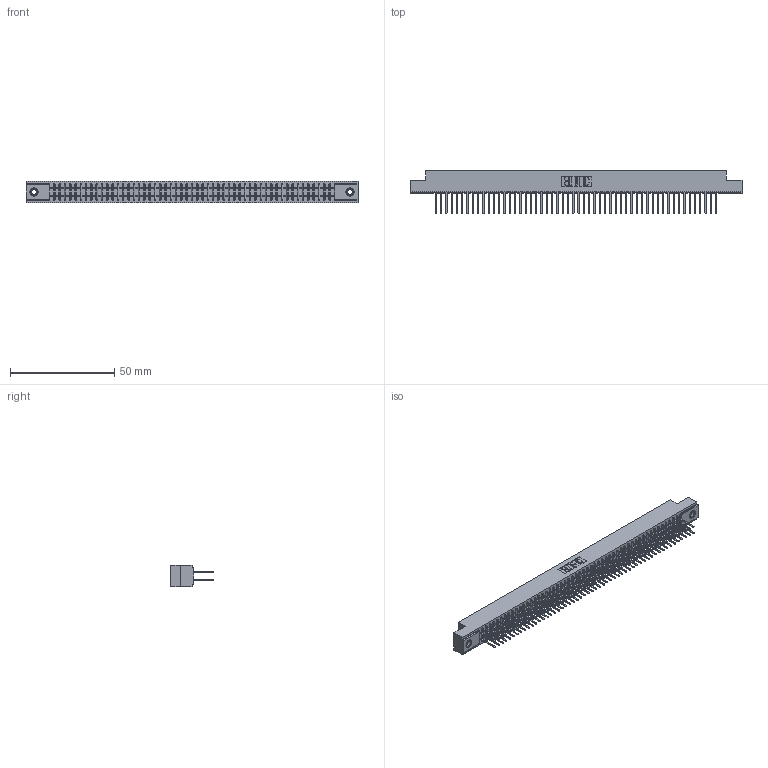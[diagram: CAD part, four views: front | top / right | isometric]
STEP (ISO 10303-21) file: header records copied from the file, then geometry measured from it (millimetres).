
FILE_DESCRIPTION (( 'STEP AP203' ), '1' );
FILE_NAME ('341-108-522-207.STEP', '2018-08-08T12:19:35', ( '' ), ( '' ), 'SwSTEP 2.0', 'SolidWorks 2016', '' );
FILE_SCHEMA (( 'CONFIG_CONTROL_DESIGN' ));
Products named in the file (4): 345-250-001_345-250-005-103; 341-108-522-207; 341 Part_.156 (3.96) Dia Mounting Holes; 341-292-001_341-292-122
Assembly tree (111 placements, depth 2):
  341-108-522-207
    341 Part_.156 (3.96) Dia Mounting Holes
    341-292-001_341-292-122  x108
    345-250-001_345-250-005-103  x2
Bounding box: 159.38 x 20.62 x 10.16 mm (x, y, z)
Volume: 11914.9 mm3; surface area: 22531.7 mm2
Topology: 111 solids, 111 shells, 7304 faces, 21134 edges, 13682 vertices
Faces by surface type: plane 4420, cylinder 2652, sphere 110, torus 110, cone 12
Entity records: 64938 total; most frequent: CARTESIAN_POINT 10777, ORIENTED_EDGE 10704, DIRECTION 10460, EDGE_CURVE 5352, VECTOR 4334, LINE 4334, VERTEX_POINT 3380, AXIS2_PLACEMENT_3D 3063
